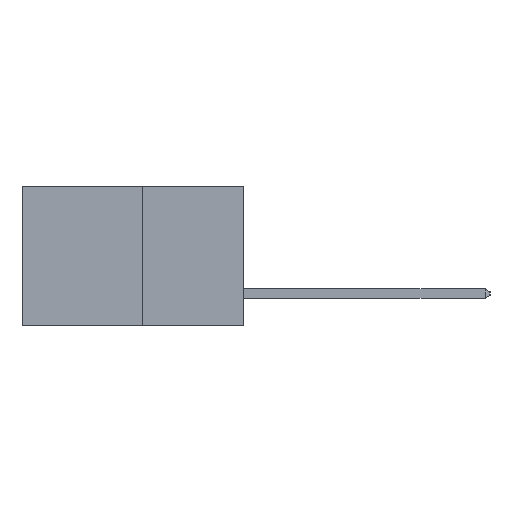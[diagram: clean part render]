
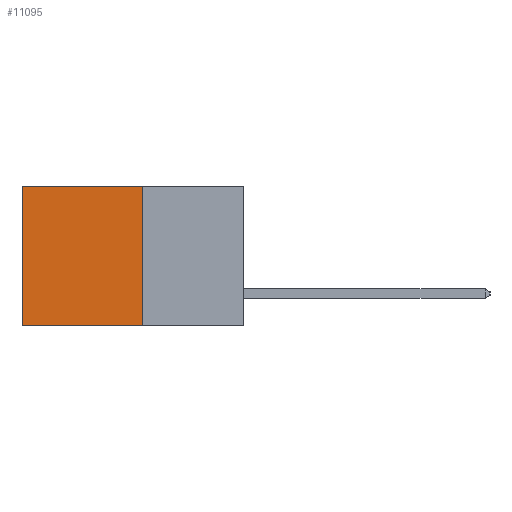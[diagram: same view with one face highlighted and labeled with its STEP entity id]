
A CAD part, left-side view. The second image highlights one B-rep face of the part: STEP entity #11095.
In plain terms, the highlighted planar face has unit normal (-1, 0, 0).
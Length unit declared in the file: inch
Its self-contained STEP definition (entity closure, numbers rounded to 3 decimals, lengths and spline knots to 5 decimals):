
#211 = ORIENTED_EDGE ( 'NONE', *, *, #2127, .F. ) ;
#301 = ORIENTED_EDGE ( 'NONE', *, *, #10525, .T. ) ;
#402 = CARTESIAN_POINT ( 'NONE',  ( 0.277, 0.59, 0. ) ) ;
#980 = LINE ( 'NONE', #7530, #5634 ) ;
#1117 = VERTEX_POINT ( 'NONE', #9139 ) ;
#1678 = CARTESIAN_POINT ( 'NONE',  ( 0.277, 0.59, -0.37 ) ) ;
#1773 = FACE_OUTER_BOUND ( 'NONE', #11243, .T. ) ;
#1788 = DIRECTION ( 'NONE',  ( 0., 0., -1. ) ) ;
#1894 = EDGE_CURVE ( 'NONE', #3762, #3551, #2770, .T. ) ;
#1997 = ORIENTED_EDGE ( 'NONE', *, *, #9124, .T. ) ;
#2070 = CARTESIAN_POINT ( 'NONE',  ( 0.277, 0.27, -0.37 ) ) ;
#2127 = EDGE_CURVE ( 'NONE', #1117, #3762, #11829, .T. ) ;
#2499 = AXIS2_PLACEMENT_3D ( 'NONE', #10023, #4708, #10932 ) ;
#2622 = DIRECTION ( 'NONE',  ( 0., 1., 0. ) ) ;
#2709 = VECTOR ( 'NONE', #2622, 39.37008 ) ;
#2770 = LINE ( 'NONE', #5942, #9359 ) ;
#3313 = LINE ( 'NONE', #7114, #2709 ) ;
#3551 = VERTEX_POINT ( 'NONE', #1678 ) ;
#3762 = VERTEX_POINT ( 'NONE', #6498 ) ;
#4708 = DIRECTION ( 'NONE',  ( 1., 0., 0. ) ) ;
#5566 = PLANE ( 'NONE',  #2499 ) ;
#5634 = VECTOR ( 'NONE', #7499, 39.37008 ) ;
#5942 = CARTESIAN_POINT ( 'NONE',  ( 0.277, 0.27, -0.37 ) ) ;
#6119 = DIRECTION ( 'NONE',  ( 0., 1., 0. ) ) ;
#6498 = CARTESIAN_POINT ( 'NONE',  ( 0.277, 0.27, -0.37 ) ) ;
#7114 = CARTESIAN_POINT ( 'NONE',  ( 0.277, 0.27, 0. ) ) ;
#7434 = VECTOR ( 'NONE', #1788, 39.37008 ) ;
#7499 = DIRECTION ( 'NONE',  ( 0., 0., -1. ) ) ;
#7530 = CARTESIAN_POINT ( 'NONE',  ( 0.277, 0.59, -0.37 ) ) ;
#9124 = EDGE_CURVE ( 'NONE', #1117, #10218, #3313, .T. ) ;
#9139 = CARTESIAN_POINT ( 'NONE',  ( 0.277, 0.27, 0. ) ) ;
#9359 = VECTOR ( 'NONE', #6119, 39.37008 ) ;
#10023 = CARTESIAN_POINT ( 'NONE',  ( 0.277, 0.27, -0.37 ) ) ;
#10218 = VERTEX_POINT ( 'NONE', #402 ) ;
#10525 = EDGE_CURVE ( 'NONE', #10218, #3551, #980, .T. ) ;
#10932 = DIRECTION ( 'NONE',  ( 0., 0., -1. ) ) ;
#11095 = ADVANCED_FACE ( 'NONE', ( #1773 ), #5566, .F. ) ;
#11243 = EDGE_LOOP ( 'NONE', ( #301, #11753, #211, #1997 ) ) ;
#11753 = ORIENTED_EDGE ( 'NONE', *, *, #1894, .F. ) ;
#11829 = LINE ( 'NONE', #2070, #7434 ) ;
